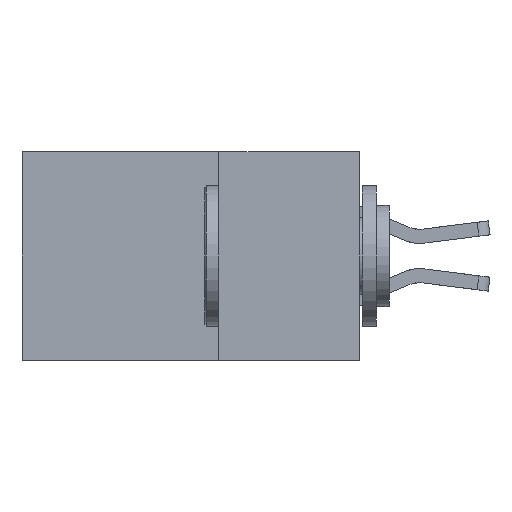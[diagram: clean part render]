
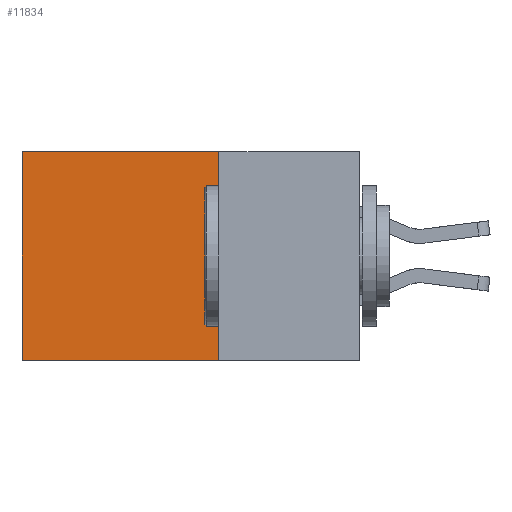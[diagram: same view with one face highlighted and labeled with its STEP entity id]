
A CAD part, left-side view. The second image highlights one B-rep face of the part: STEP entity #11834.
In plain terms, the highlighted planar face has unit normal (-1, 0, 0).
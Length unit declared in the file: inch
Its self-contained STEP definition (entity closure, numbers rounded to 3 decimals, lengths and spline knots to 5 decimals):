
#435 = VERTEX_POINT ( 'NONE', #14966 ) ;
#777 = CARTESIAN_POINT ( 'NONE',  ( 0.2875, 0.25, 0. ) ) ;
#1202 = VERTEX_POINT ( 'NONE', #6260 ) ;
#1456 = LINE ( 'NONE', #3101, #13625 ) ;
#1810 = LINE ( 'NONE', #6706, #11066 ) ;
#2151 = DIRECTION ( 'NONE',  ( 0., 1., 0. ) ) ;
#2558 = PLANE ( 'NONE',  #7111 ) ;
#2608 = DIRECTION ( 'NONE',  ( 0., 0., -1. ) ) ;
#3010 = CARTESIAN_POINT ( 'NONE',  ( 0.2875, 0.6, -0.37 ) ) ;
#3024 = ORIENTED_EDGE ( 'NONE', *, *, #7952, .F. ) ;
#3101 = CARTESIAN_POINT ( 'NONE',  ( 0.2875, 0.6, 0. ) ) ;
#4411 = LINE ( 'NONE', #5010, #9130 ) ;
#5010 = CARTESIAN_POINT ( 'NONE',  ( 0.2875, 0.25, 0. ) ) ;
#5303 = ORIENTED_EDGE ( 'NONE', *, *, #13165, .F. ) ;
#5938 = VERTEX_POINT ( 'NONE', #11132 ) ;
#6260 = CARTESIAN_POINT ( 'NONE',  ( 0.2875, 0.25, 0. ) ) ;
#6706 = CARTESIAN_POINT ( 'NONE',  ( 0.2875, 0.25, -0.37 ) ) ;
#7111 = AXIS2_PLACEMENT_3D ( 'NONE', #13066, #13015, #2608 ) ;
#7448 = EDGE_CURVE ( 'NONE', #435, #9255, #1456, .T. ) ;
#7952 = EDGE_CURVE ( 'NONE', #5938, #9255, #1810, .T. ) ;
#8929 = VECTOR ( 'NONE', #9076, 39.37008 ) ;
#9076 = DIRECTION ( 'NONE',  ( 0., 0., -1. ) ) ;
#9130 = VECTOR ( 'NONE', #13179, 39.37008 ) ;
#9255 = VERTEX_POINT ( 'NONE', #3010 ) ;
#10243 = FACE_OUTER_BOUND ( 'NONE', #11534, .T. ) ;
#11066 = VECTOR ( 'NONE', #2151, 39.37008 ) ;
#11132 = CARTESIAN_POINT ( 'NONE',  ( 0.2875, 0.25, -0.37 ) ) ;
#11194 = ORIENTED_EDGE ( 'NONE', *, *, #12844, .T. ) ;
#11400 = DIRECTION ( 'NONE',  ( 0., 0., -1. ) ) ;
#11534 = EDGE_LOOP ( 'NONE', ( #14231, #3024, #5303, #11194 ) ) ;
#11834 = ADVANCED_FACE ( 'NONE', ( #10243 ), #2558, .F. ) ;
#12844 = EDGE_CURVE ( 'NONE', #1202, #435, #4411, .T. ) ;
#13015 = DIRECTION ( 'NONE',  ( 1., 0., 0. ) ) ;
#13066 = CARTESIAN_POINT ( 'NONE',  ( 0.2875, 0.25, 0. ) ) ;
#13165 = EDGE_CURVE ( 'NONE', #1202, #5938, #13642, .T. ) ;
#13179 = DIRECTION ( 'NONE',  ( 0., 1., 0. ) ) ;
#13625 = VECTOR ( 'NONE', #11400, 39.37008 ) ;
#13642 = LINE ( 'NONE', #777, #8929 ) ;
#14231 = ORIENTED_EDGE ( 'NONE', *, *, #7448, .T. ) ;
#14966 = CARTESIAN_POINT ( 'NONE',  ( 0.2875, 0.6, 0. ) ) ;
